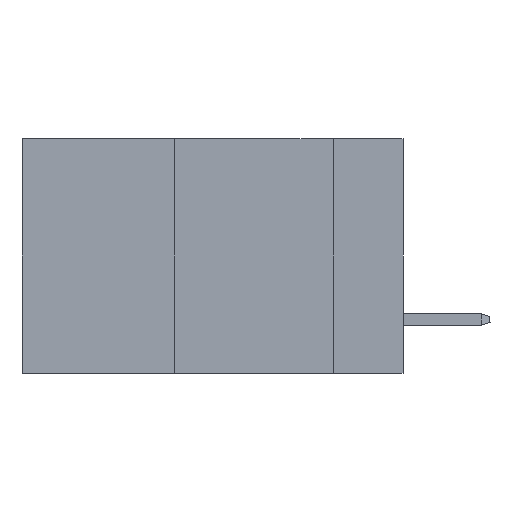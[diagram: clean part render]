
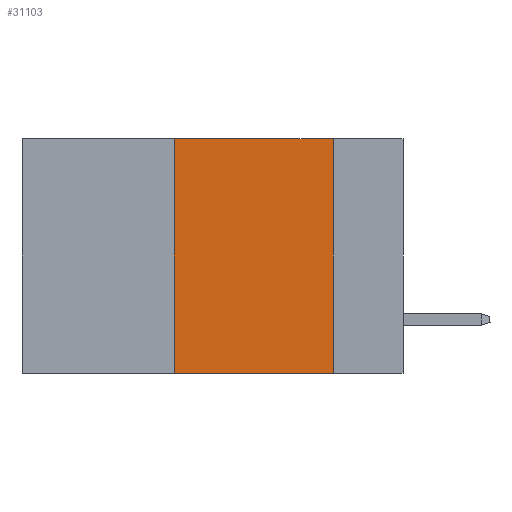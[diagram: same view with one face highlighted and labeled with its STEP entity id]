
A CAD part, left-side view. The second image highlights one B-rep face of the part: STEP entity #31103.
In plain terms, the highlighted planar face has unit normal (-1, 0, 0).
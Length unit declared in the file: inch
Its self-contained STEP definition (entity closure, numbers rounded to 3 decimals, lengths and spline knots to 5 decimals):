
#188 = VECTOR ( 'NONE', #20719, 39.37008 ) ;
#457 = CARTESIAN_POINT ( 'NONE',  ( 0., 0.11, 0. ) ) ;
#921 = VERTEX_POINT ( 'NONE', #25395 ) ;
#2110 = VERTEX_POINT ( 'NONE', #3847 ) ;
#3454 = EDGE_CURVE ( 'NONE', #921, #9269, #25621, .T. ) ;
#3588 = PLANE ( 'NONE',  #17389 ) ;
#3847 = CARTESIAN_POINT ( 'NONE',  ( 0., 0.11, -0.37 ) ) ;
#4004 = DIRECTION ( 'NONE',  ( 0., 0., 1. ) ) ;
#4592 = VECTOR ( 'NONE', #4004, 39.37008 ) ;
#5701 = CARTESIAN_POINT ( 'NONE',  ( 0., 0.36, 0. ) ) ;
#6068 = CARTESIAN_POINT ( 'NONE',  ( 0., 0.36, 0. ) ) ;
#6189 = CARTESIAN_POINT ( 'NONE',  ( 0., 0.11, 0. ) ) ;
#6353 = LINE ( 'NONE', #6189, #20251 ) ;
#8494 = CARTESIAN_POINT ( 'NONE',  ( 0., 0.6, 0. ) ) ;
#8932 = LINE ( 'NONE', #27689, #15254 ) ;
#9269 = VERTEX_POINT ( 'NONE', #5701 ) ;
#11413 = CARTESIAN_POINT ( 'NONE',  ( 0., 0.6, 0. ) ) ;
#13076 = FACE_OUTER_BOUND ( 'NONE', #16949, .T. ) ;
#14952 = ORIENTED_EDGE ( 'NONE', *, *, #22678, .T. ) ;
#15254 = VECTOR ( 'NONE', #20749, 39.37008 ) ;
#16949 = EDGE_LOOP ( 'NONE', ( #25642, #23627, #22403, #14952 ) ) ;
#17389 = AXIS2_PLACEMENT_3D ( 'NONE', #8494, #29934, #27727 ) ;
#20251 = VECTOR ( 'NONE', #25736, 39.37008 ) ;
#20490 = VERTEX_POINT ( 'NONE', #457 ) ;
#20719 = DIRECTION ( 'NONE',  ( 0., -1., 0. ) ) ;
#20749 = DIRECTION ( 'NONE',  ( 0., -1., 0. ) ) ;
#21522 = EDGE_CURVE ( 'NONE', #20490, #2110, #6353, .T. ) ;
#22403 = ORIENTED_EDGE ( 'NONE', *, *, #3454, .F. ) ;
#22678 = EDGE_CURVE ( 'NONE', #921, #2110, #8932, .T. ) ;
#23627 = ORIENTED_EDGE ( 'NONE', *, *, #24471, .F. ) ;
#24471 = EDGE_CURVE ( 'NONE', #9269, #20490, #27656, .T. ) ;
#25395 = CARTESIAN_POINT ( 'NONE',  ( 0., 0.36, -0.37 ) ) ;
#25621 = LINE ( 'NONE', #6068, #4592 ) ;
#25642 = ORIENTED_EDGE ( 'NONE', *, *, #21522, .F. ) ;
#25736 = DIRECTION ( 'NONE',  ( 0., 0., -1. ) ) ;
#27656 = LINE ( 'NONE', #11413, #188 ) ;
#27689 = CARTESIAN_POINT ( 'NONE',  ( 0., 0.6, -0.37 ) ) ;
#27727 = DIRECTION ( 'NONE',  ( 0., 0., -1. ) ) ;
#29934 = DIRECTION ( 'NONE',  ( 1., 0., 0. ) ) ;
#31103 = ADVANCED_FACE ( 'NONE', ( #13076 ), #3588, .F. ) ;
